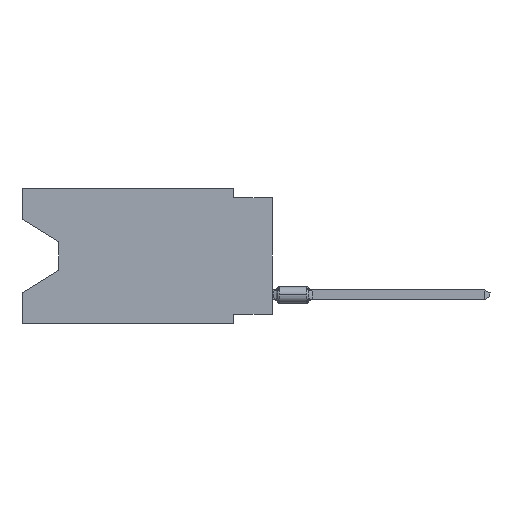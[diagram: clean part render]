
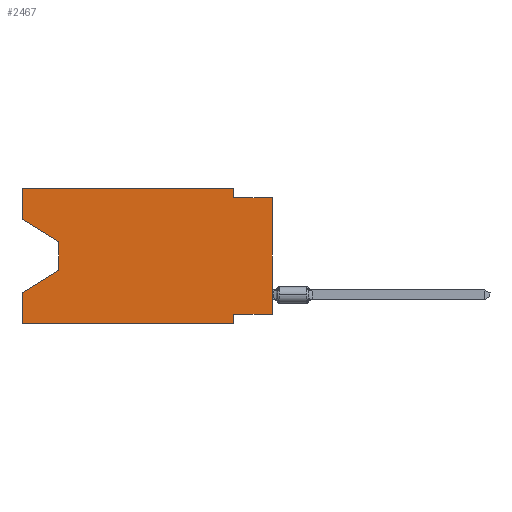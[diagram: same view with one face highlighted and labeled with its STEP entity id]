
A CAD part, left-side view. The second image highlights one B-rep face of the part: STEP entity #2467.
In plain terms, the highlighted planar face has unit normal (-1, 0, 0).
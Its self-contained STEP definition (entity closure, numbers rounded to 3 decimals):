
#71 = AXIS2_PLACEMENT_3D ( 'NONE', #39101, #23620, #43349 ) ;
#368 = CARTESIAN_POINT ( 'NONE',  ( 0., 2.54, -8.255 ) ) ;
#1167 = ORIENTED_EDGE ( 'NONE', *, *, #18133, .F. ) ;
#1443 = VERTEX_POINT ( 'NONE', #51271 ) ;
#1712 = ORIENTED_EDGE ( 'NONE', *, *, #44666, .F. ) ;
#1833 = DIRECTION ( 'NONE',  ( 0., -0.855, -0.519 ) ) ;
#2467 = ADVANCED_FACE ( 'NONE', ( #2839 ), #47342, .F. ) ;
#2635 = CARTESIAN_POINT ( 'NONE',  ( 0., 16.383, -6.852 ) ) ;
#2686 = DIRECTION ( 'NONE',  ( 0., 0., -1. ) ) ;
#2839 = FACE_OUTER_BOUND ( 'NONE', #42290, .T. ) ;
#6589 = DIRECTION ( 'NONE',  ( 0., 0.855, -0.519 ) ) ;
#6983 = VERTEX_POINT ( 'NONE', #12898 ) ;
#7772 = EDGE_CURVE ( 'NONE', #1443, #35683, #13605, .T. ) ;
#9835 = VECTOR ( 'NONE', #19322, 1000. ) ;
#11307 = CARTESIAN_POINT ( 'NONE',  ( 0., 16.383, 0. ) ) ;
#12059 = CARTESIAN_POINT ( 'NONE',  ( 0., 2.54, 0. ) ) ;
#12503 = VECTOR ( 'NONE', #49999, 1000. ) ;
#12898 = CARTESIAN_POINT ( 'NONE',  ( 0., 2.54, -8.89 ) ) ;
#13422 = CARTESIAN_POINT ( 'NONE',  ( 0., 16.383, 0. ) ) ;
#13605 = LINE ( 'NONE', #17342, #36840 ) ;
#13963 = LINE ( 'NONE', #38740, #29344 ) ;
#14081 = LINE ( 'NONE', #38361, #42537 ) ;
#14556 = ORIENTED_EDGE ( 'NONE', *, *, #42706, .T. ) ;
#15325 = DIRECTION ( 'NONE',  ( 0., -1., 0. ) ) ;
#15977 = VERTEX_POINT ( 'NONE', #38694 ) ;
#16060 = VECTOR ( 'NONE', #47347, 1000. ) ;
#17342 = CARTESIAN_POINT ( 'NONE',  ( 0., 0., 0. ) ) ;
#17498 = LINE ( 'NONE', #33759, #12503 ) ;
#17695 = DIRECTION ( 'NONE',  ( 0., 0., -1. ) ) ;
#18065 = EDGE_CURVE ( 'NONE', #29178, #6983, #34859, .T. ) ;
#18070 = VECTOR ( 'NONE', #15325, 1000. ) ;
#18133 = EDGE_CURVE ( 'NONE', #29240, #44652, #26588, .T. ) ;
#19322 = DIRECTION ( 'NONE',  ( 0., 1., 0. ) ) ;
#19326 = DIRECTION ( 'NONE',  ( 0., 0., 1. ) ) ;
#19882 = ORIENTED_EDGE ( 'NONE', *, *, #21838, .F. ) ;
#19994 = CARTESIAN_POINT ( 'NONE',  ( 0., 13.97, -3.505 ) ) ;
#21426 = EDGE_CURVE ( 'NONE', #29240, #50487, #14081, .T. ) ;
#21838 = EDGE_CURVE ( 'NONE', #31753, #41332, #51835, .T. ) ;
#22306 = ORIENTED_EDGE ( 'NONE', *, *, #43770, .T. ) ;
#22354 = CARTESIAN_POINT ( 'NONE',  ( 0., 16.383, -8.89 ) ) ;
#22589 = CARTESIAN_POINT ( 'NONE',  ( 0., 16.383, 0. ) ) ;
#23620 = DIRECTION ( 'NONE',  ( 1., 0., 0. ) ) ;
#26290 = CARTESIAN_POINT ( 'NONE',  ( 0., 0., -0.635 ) ) ;
#26352 = DIRECTION ( 'NONE',  ( 0., -1., 0. ) ) ;
#26588 = LINE ( 'NONE', #22589, #36501 ) ;
#27613 = ORIENTED_EDGE ( 'NONE', *, *, #18065, .F. ) ;
#27836 = CARTESIAN_POINT ( 'NONE',  ( 0., 0., -8.255 ) ) ;
#28680 = VECTOR ( 'NONE', #6589, 1000. ) ;
#29178 = VERTEX_POINT ( 'NONE', #368 ) ;
#29240 = VERTEX_POINT ( 'NONE', #50474 ) ;
#29344 = VECTOR ( 'NONE', #17695, 1000. ) ;
#30330 = LINE ( 'NONE', #22354, #37812 ) ;
#30856 = EDGE_CURVE ( 'NONE', #1443, #29178, #48352, .T. ) ;
#31461 = LINE ( 'NONE', #19994, #50472 ) ;
#31619 = ORIENTED_EDGE ( 'NONE', *, *, #21426, .T. ) ;
#31753 = VERTEX_POINT ( 'NONE', #47897 ) ;
#31877 = EDGE_CURVE ( 'NONE', #44652, #52239, #17498, .T. ) ;
#33059 = VERTEX_POINT ( 'NONE', #47787 ) ;
#33759 = CARTESIAN_POINT ( 'NONE',  ( 0., 16.383, 0. ) ) ;
#34859 = LINE ( 'NONE', #43354, #16060 ) ;
#35112 = DIRECTION ( 'NONE',  ( 0., 0., 1. ) ) ;
#35200 = EDGE_CURVE ( 'NONE', #33059, #41332, #51125, .T. ) ;
#35683 = VERTEX_POINT ( 'NONE', #26290 ) ;
#36501 = VECTOR ( 'NONE', #35112, 1000. ) ;
#36840 = VECTOR ( 'NONE', #49842, 1000. ) ;
#37251 = CARTESIAN_POINT ( 'NONE',  ( 0., 13.97, -3.505 ) ) ;
#37812 = VECTOR ( 'NONE', #26352, 1000. ) ;
#38090 = CARTESIAN_POINT ( 'NONE',  ( 0., 13.97, -5.385 ) ) ;
#38361 = CARTESIAN_POINT ( 'NONE',  ( 0., 16.383, -2.038 ) ) ;
#38694 = CARTESIAN_POINT ( 'NONE',  ( 0., 2.54, -0.635 ) ) ;
#38740 = CARTESIAN_POINT ( 'NONE',  ( 0., 2.54, 0. ) ) ;
#39101 = CARTESIAN_POINT ( 'NONE',  ( 0., 16.383, 0. ) ) ;
#41332 = VERTEX_POINT ( 'NONE', #2635 ) ;
#41363 = ORIENTED_EDGE ( 'NONE', *, *, #31877, .F. ) ;
#41821 = EDGE_CURVE ( 'NONE', #15977, #35683, #48875, .T. ) ;
#42290 = EDGE_LOOP ( 'NONE', ( #31619, #14556, #48332, #19882, #22306, #27613, #51914, #51519, #46544, #1712, #41363, #1167 ) ) ;
#42537 = VECTOR ( 'NONE', #1833, 1000. ) ;
#42706 = EDGE_CURVE ( 'NONE', #50487, #33059, #31461, .T. ) ;
#43349 = DIRECTION ( 'NONE',  ( 0., 0., -1. ) ) ;
#43354 = CARTESIAN_POINT ( 'NONE',  ( 0., 2.54, -8.89 ) ) ;
#43770 = EDGE_CURVE ( 'NONE', #31753, #6983, #30330, .T. ) ;
#44652 = VERTEX_POINT ( 'NONE', #13422 ) ;
#44666 = EDGE_CURVE ( 'NONE', #52239, #15977, #13963, .T. ) ;
#46544 = ORIENTED_EDGE ( 'NONE', *, *, #41821, .F. ) ;
#47342 = PLANE ( 'NONE',  #71 ) ;
#47347 = DIRECTION ( 'NONE',  ( 0., 0., -1. ) ) ;
#47787 = CARTESIAN_POINT ( 'NONE',  ( 0., 13.97, -5.385 ) ) ;
#47897 = CARTESIAN_POINT ( 'NONE',  ( 0., 16.383, -8.89 ) ) ;
#48332 = ORIENTED_EDGE ( 'NONE', *, *, #35200, .T. ) ;
#48352 = LINE ( 'NONE', #27836, #9835 ) ;
#48875 = LINE ( 'NONE', #52093, #18070 ) ;
#49842 = DIRECTION ( 'NONE',  ( 0., 0., 1. ) ) ;
#49999 = DIRECTION ( 'NONE',  ( 0., -1., 0. ) ) ;
#50472 = VECTOR ( 'NONE', #2686, 1000. ) ;
#50474 = CARTESIAN_POINT ( 'NONE',  ( 0., 16.383, -2.038 ) ) ;
#50487 = VERTEX_POINT ( 'NONE', #37251 ) ;
#51125 = LINE ( 'NONE', #38090, #28680 ) ;
#51271 = CARTESIAN_POINT ( 'NONE',  ( 0., 0., -8.255 ) ) ;
#51519 = ORIENTED_EDGE ( 'NONE', *, *, #7772, .T. ) ;
#51835 = LINE ( 'NONE', #11307, #52648 ) ;
#51914 = ORIENTED_EDGE ( 'NONE', *, *, #30856, .F. ) ;
#52093 = CARTESIAN_POINT ( 'NONE',  ( 0., 0., -0.635 ) ) ;
#52239 = VERTEX_POINT ( 'NONE', #12059 ) ;
#52648 = VECTOR ( 'NONE', #19326, 1000. ) ;
